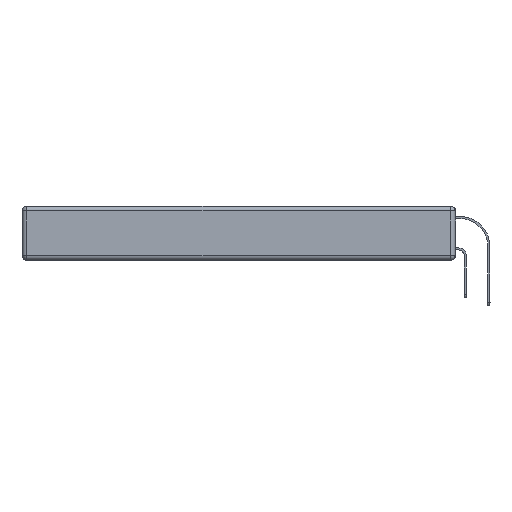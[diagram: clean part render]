
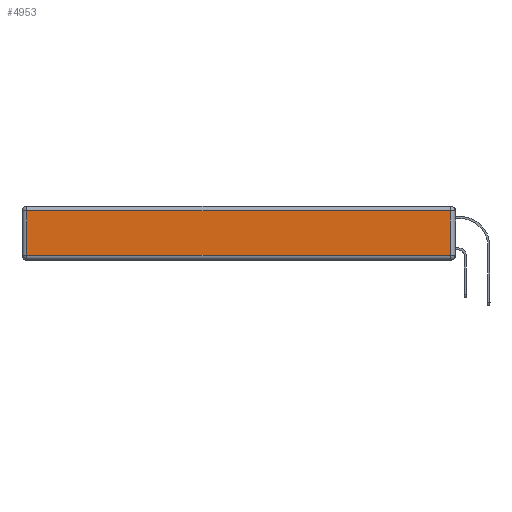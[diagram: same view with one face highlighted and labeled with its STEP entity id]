
A CAD part, left-side view. The second image highlights one B-rep face of the part: STEP entity #4953.
In plain terms, the highlighted planar face has unit normal (-1, 0, 0).
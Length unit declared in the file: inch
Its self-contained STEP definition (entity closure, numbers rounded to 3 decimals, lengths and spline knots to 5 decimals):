
#204 = ORIENTED_EDGE ( 'NONE', *, *, #293, .T. ) ;
#268 = VECTOR ( 'NONE', #13982, 39.37008 ) ;
#293 = EDGE_CURVE ( 'NONE', #1514, #10063, #15031, .T. ) ;
#1514 = VERTEX_POINT ( 'NONE', #21561 ) ;
#4461 = LINE ( 'NONE', #9079, #7251 ) ;
#4953 = ADVANCED_FACE ( 'NONE', ( #28456 ), #8126, .T. ) ;
#5900 = DIRECTION ( 'NONE',  ( -1., 0., 0. ) ) ;
#6442 = CARTESIAN_POINT ( 'NONE',  ( 0., 2.72, -0.03 ) ) ;
#7251 = VECTOR ( 'NONE', #28826, 39.37008 ) ;
#8126 = PLANE ( 'NONE',  #14192 ) ;
#8438 = ORIENTED_EDGE ( 'NONE', *, *, #25155, .T. ) ;
#9079 = CARTESIAN_POINT ( 'NONE',  ( 0., 0., -0.313 ) ) ;
#10063 = VERTEX_POINT ( 'NONE', #6442 ) ;
#10609 = EDGE_CURVE ( 'NONE', #13770, #14623, #4461, .T. ) ;
#12658 = CARTESIAN_POINT ( 'NONE',  ( 0., 2.75, -0.03 ) ) ;
#12735 = DIRECTION ( 'NONE',  ( 0., 0., 1. ) ) ;
#13770 = VERTEX_POINT ( 'NONE', #24984 ) ;
#13982 = DIRECTION ( 'NONE',  ( 0., 0., 1. ) ) ;
#14192 = AXIS2_PLACEMENT_3D ( 'NONE', #26229, #5900, #12735 ) ;
#14219 = ORIENTED_EDGE ( 'NONE', *, *, #10609, .T. ) ;
#14623 = VERTEX_POINT ( 'NONE', #20445 ) ;
#15031 = LINE ( 'NONE', #12658, #21910 ) ;
#16453 = EDGE_LOOP ( 'NONE', ( #14219, #8438, #204, #20081 ) ) ;
#18454 = LINE ( 'NONE', #20514, #268 ) ;
#20081 = ORIENTED_EDGE ( 'NONE', *, *, #20169, .T. ) ;
#20169 = EDGE_CURVE ( 'NONE', #10063, #13770, #26968, .T. ) ;
#20445 = CARTESIAN_POINT ( 'NONE',  ( 0., 0.03, -0.313 ) ) ;
#20514 = CARTESIAN_POINT ( 'NONE',  ( 0., 0.03, -0.343 ) ) ;
#21561 = CARTESIAN_POINT ( 'NONE',  ( 0., 0.03, -0.03 ) ) ;
#21910 = VECTOR ( 'NONE', #26600, 39.37008 ) ;
#24421 = CARTESIAN_POINT ( 'NONE',  ( 0., 2.72, -0.343 ) ) ;
#24482 = VECTOR ( 'NONE', #24866, 39.37008 ) ;
#24866 = DIRECTION ( 'NONE',  ( 0., 0., -1. ) ) ;
#24984 = CARTESIAN_POINT ( 'NONE',  ( 0., 2.72, -0.313 ) ) ;
#25155 = EDGE_CURVE ( 'NONE', #14623, #1514, #18454, .T. ) ;
#26229 = CARTESIAN_POINT ( 'NONE',  ( 0., 0., -0.343 ) ) ;
#26600 = DIRECTION ( 'NONE',  ( 0., 1., 0. ) ) ;
#26968 = LINE ( 'NONE', #24421, #24482 ) ;
#28456 = FACE_OUTER_BOUND ( 'NONE', #16453, .T. ) ;
#28826 = DIRECTION ( 'NONE',  ( 0., -1., 0. ) ) ;
